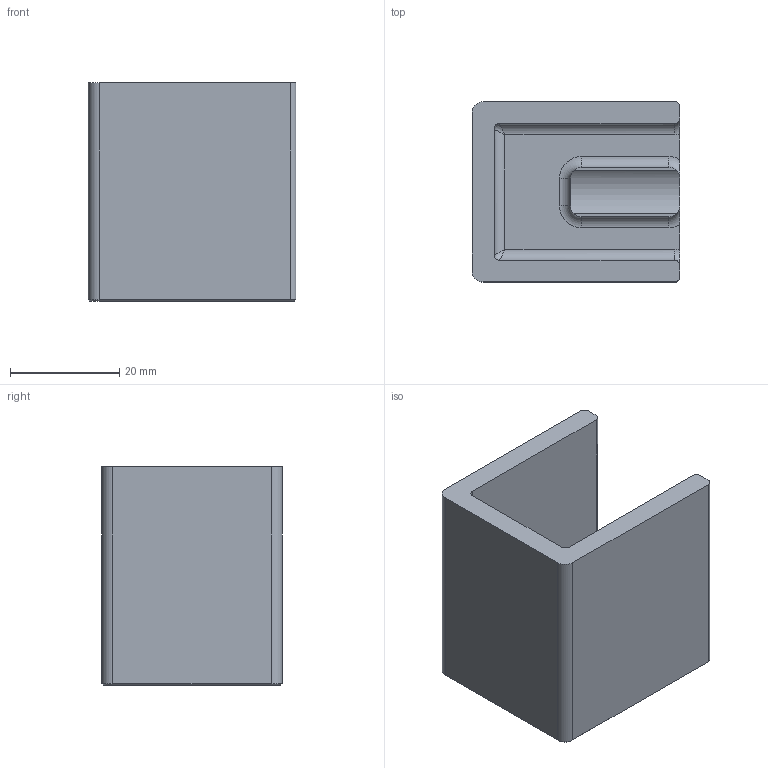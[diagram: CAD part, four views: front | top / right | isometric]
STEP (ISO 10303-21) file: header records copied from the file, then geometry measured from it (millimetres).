
FILE_DESCRIPTION(/* description */ (''),/* implementation_level */ '2;1');
FILE_NAME(/* name */ 'aics_magazine_loader.step',/* time_stamp */ '2022-10-27T02:01:12+13:00',/* author */ (''),/* organization */ (''),/* preprocessor_version */ 'ST-DEVELOPER v19.2',/* originating_system */ 'Autodesk Translation Framework v11.17.0.187',/* authorisation */ '');
FILE_SCHEMA (('AUTOMOTIVE_DESIGN { 1 0 10303 214 3 1 1 }'));
Length unit declared in the file: millimetre
Products named in the file (1): aics_magazine_loader
Bounding box: 38 x 33 x 40 mm (x, y, z)
Volume: 21721.3 mm3; surface area: 11033.2 mm2
Topology: 1 solids, 1 shells, 50 faces, 124 edges, 74 vertices
Faces by surface type: plane 19, cylinder 19, torus 6, cone 4, bspline 2
Entity records: 1591 total; most frequent: CARTESIAN_POINT 369, DIRECTION 260, ORIENTED_EDGE 244, EDGE_CURVE 122, AXIS2_PLACEMENT_3D 97, VERTEX_POINT 74, LINE 66, VECTOR 66
